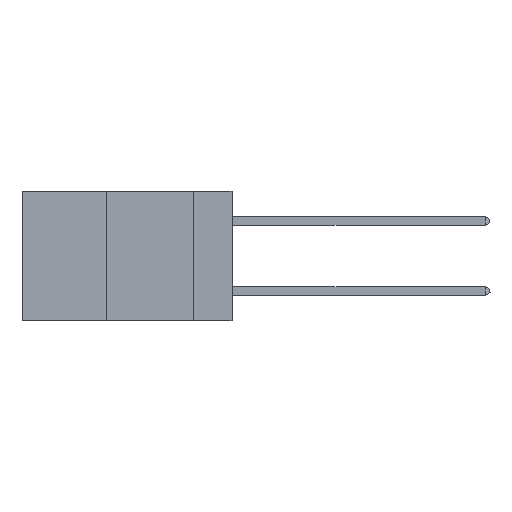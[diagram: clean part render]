
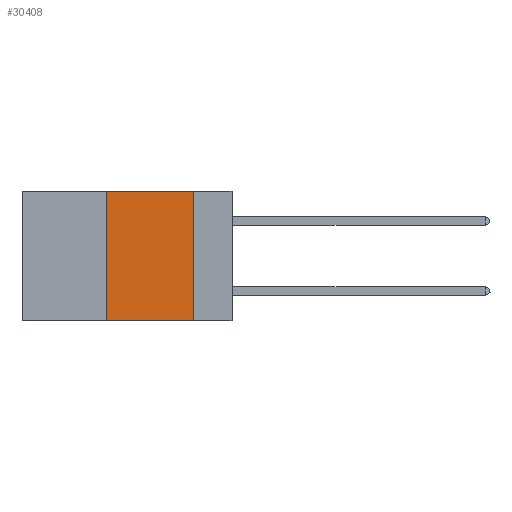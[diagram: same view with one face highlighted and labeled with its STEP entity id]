
A CAD part, left-side view. The second image highlights one B-rep face of the part: STEP entity #30408.
In plain terms, the highlighted planar face has unit normal (-1, 0, 0).
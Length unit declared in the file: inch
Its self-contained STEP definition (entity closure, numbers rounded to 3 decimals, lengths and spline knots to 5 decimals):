
#1849 = ORIENTED_EDGE ( 'NONE', *, *, #10268, .T. ) ;
#3692 = ORIENTED_EDGE ( 'NONE', *, *, #21190, .F. ) ;
#4753 = FACE_OUTER_BOUND ( 'NONE', #22074, .T. ) ;
#4918 = DIRECTION ( 'NONE',  ( 1., 0., 0. ) ) ;
#5091 = CARTESIAN_POINT ( 'NONE',  ( 0., 0.6, 0. ) ) ;
#5336 = DIRECTION ( 'NONE',  ( 0., 0., -1. ) ) ;
#6969 = CARTESIAN_POINT ( 'NONE',  ( 0., 0.6, -0.37 ) ) ;
#7309 = LINE ( 'NONE', #6969, #25814 ) ;
#9979 = LINE ( 'NONE', #23028, #19983 ) ;
#10268 = EDGE_CURVE ( 'NONE', #17622, #26221, #7309, .T. ) ;
#11129 = EDGE_CURVE ( 'NONE', #17622, #29578, #9979, .T. ) ;
#11130 = DIRECTION ( 'NONE',  ( 0., -1., 0. ) ) ;
#11184 = VECTOR ( 'NONE', #11130, 39.37008 ) ;
#11446 = AXIS2_PLACEMENT_3D ( 'NONE', #5091, #4918, #30071 ) ;
#12121 = DIRECTION ( 'NONE',  ( 0., -1., 0. ) ) ;
#12415 = CARTESIAN_POINT ( 'NONE',  ( 0., 0.36, -0.37 ) ) ;
#14307 = CARTESIAN_POINT ( 'NONE',  ( 0., 0.36, 0. ) ) ;
#15608 = EDGE_CURVE ( 'NONE', #29578, #25966, #28509, .T. ) ;
#17622 = VERTEX_POINT ( 'NONE', #12415 ) ;
#18054 = DIRECTION ( 'NONE',  ( 0., 0., 1. ) ) ;
#18063 = LINE ( 'NONE', #28485, #19637 ) ;
#18817 = CARTESIAN_POINT ( 'NONE',  ( 0., 0.11, -0.37 ) ) ;
#19637 = VECTOR ( 'NONE', #5336, 39.37008 ) ;
#19983 = VECTOR ( 'NONE', #18054, 39.37008 ) ;
#21190 = EDGE_CURVE ( 'NONE', #25966, #26221, #18063, .T. ) ;
#22074 = EDGE_LOOP ( 'NONE', ( #3692, #29932, #22407, #1849 ) ) ;
#22407 = ORIENTED_EDGE ( 'NONE', *, *, #11129, .F. ) ;
#23028 = CARTESIAN_POINT ( 'NONE',  ( 0., 0.36, 0. ) ) ;
#25814 = VECTOR ( 'NONE', #12121, 39.37008 ) ;
#25966 = VERTEX_POINT ( 'NONE', #31644 ) ;
#26185 = CARTESIAN_POINT ( 'NONE',  ( 0., 0.6, 0. ) ) ;
#26221 = VERTEX_POINT ( 'NONE', #18817 ) ;
#27095 = PLANE ( 'NONE',  #11446 ) ;
#28485 = CARTESIAN_POINT ( 'NONE',  ( 0., 0.11, 0. ) ) ;
#28509 = LINE ( 'NONE', #26185, #11184 ) ;
#29578 = VERTEX_POINT ( 'NONE', #14307 ) ;
#29932 = ORIENTED_EDGE ( 'NONE', *, *, #15608, .F. ) ;
#30071 = DIRECTION ( 'NONE',  ( 0., 0., -1. ) ) ;
#30408 = ADVANCED_FACE ( 'NONE', ( #4753 ), #27095, .F. ) ;
#31644 = CARTESIAN_POINT ( 'NONE',  ( 0., 0.11, 0. ) ) ;
